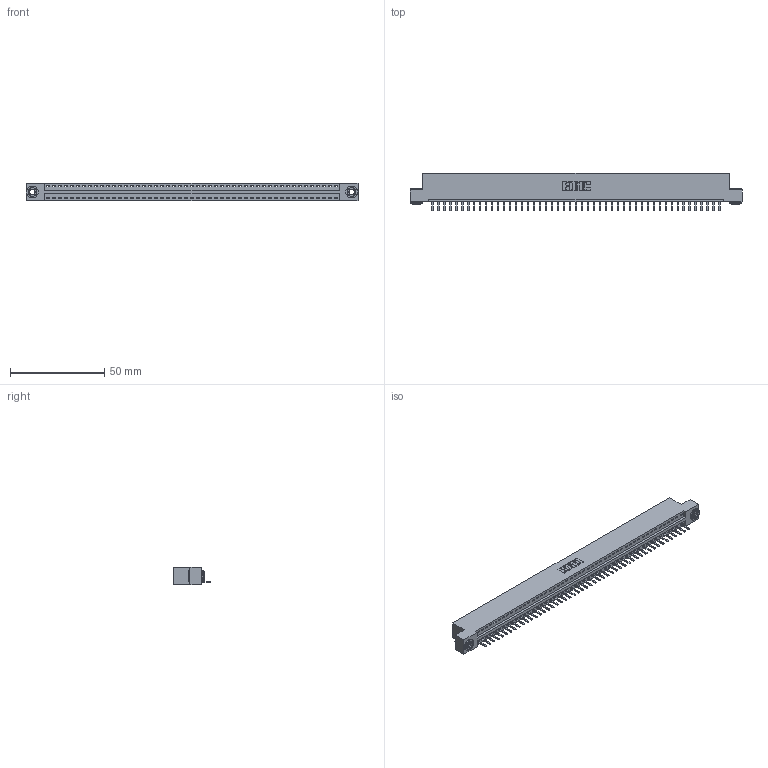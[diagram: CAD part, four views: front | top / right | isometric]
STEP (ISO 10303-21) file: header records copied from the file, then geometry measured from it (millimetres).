
FILE_DESCRIPTION (( 'STEP AP203' ), '1' );
FILE_NAME ('346-049-520-103.STEP', '2022-05-10T00:43:48', ( '' ), ( '' ), 'SwSTEP 2.0', 'SolidWorks 2020', '' );
FILE_SCHEMA (( 'CONFIG_CONTROL_DESIGN' ));
Length unit declared in the file: inch
Products named in the file (4): 345-250-002_345-250-002-102; 346-049-520-103; 345-292-001_345-293-120; 346 Part_Flush Mounting Lugs - 0.156 Dia-TH
Assembly tree (52 placements, depth 2):
  346-049-520-103
    346 Part_Flush Mounting Lugs - 0.156 Dia-TH
    345-292-001_345-293-120  x49
    345-250-002_345-250-002-102  x2
Bounding box: 176.15 x 20.02 x 9.4 mm (x, y, z)
Volume: 16769.9 mm3; surface area: 20816.7 mm2
Topology: 52 solids, 52 shells, 3212 faces, 9457 edges, 6170 vertices
Faces by surface type: plane 2158, cylinder 1046, cone 8
Entity records: 30648 total; most frequent: CARTESIAN_POINT 5244, ORIENTED_EDGE 5206, DIRECTION 4635, EDGE_CURVE 2603, VECTOR 2247, LINE 2247, VERTEX_POINT 1730, AXIS2_PLACEMENT_3D 1194
